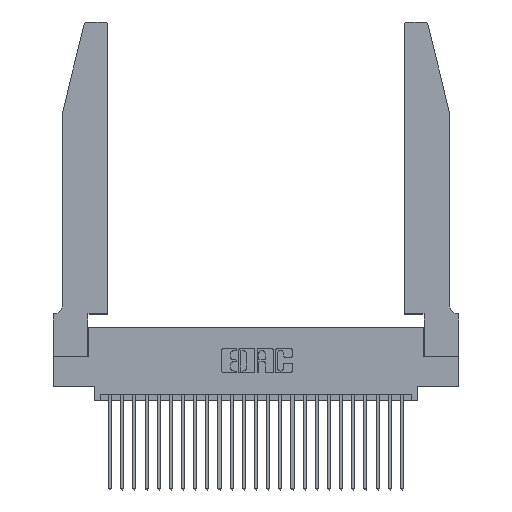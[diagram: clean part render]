
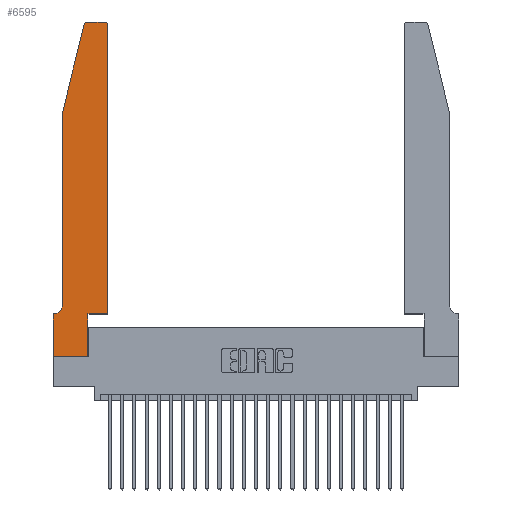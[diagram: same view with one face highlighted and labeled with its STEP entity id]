
A CAD part, top view. The second image highlights one B-rep face of the part: STEP entity #6595.
In plain terms, the highlighted planar face has unit normal (0, 0, 1).
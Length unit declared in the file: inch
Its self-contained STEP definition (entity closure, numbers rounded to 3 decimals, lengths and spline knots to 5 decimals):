
#409 = DIRECTION ( 'NONE',  ( 0., -1., 0. ) ) ;
#689 = AXIS2_PLACEMENT_3D ( 'NONE', #11758, #26268, #13857 ) ;
#794 = CARTESIAN_POINT ( 'NONE',  ( 0.0755, 2., 0.37 ) ) ;
#1211 = ORIENTED_EDGE ( 'NONE', *, *, #2643, .T. ) ;
#1948 = DIRECTION ( 'NONE',  ( 0., -1., 0. ) ) ;
#1983 = FACE_OUTER_BOUND ( 'NONE', #3229, .T. ) ;
#2109 = VERTEX_POINT ( 'NONE', #17667 ) ;
#2643 = EDGE_CURVE ( 'NONE', #11408, #11987, #24887, .T. ) ;
#2782 = AXIS2_PLACEMENT_3D ( 'NONE', #10301, #24837, #12374 ) ;
#2885 = VERTEX_POINT ( 'NONE', #21233 ) ;
#3229 = EDGE_LOOP ( 'NONE', ( #14582, #19071, #8017, #21854, #19484, #22160, #19364, #4074, #26821, #16894, #23213, #1211 ) ) ;
#3261 = AXIS2_PLACEMENT_3D ( 'NONE', #9698, #24244, #11782 ) ;
#3328 = DIRECTION ( 'NONE',  ( 0., 1., 0. ) ) ;
#4070 = CARTESIAN_POINT ( 'NONE',  ( 0.4505, 0.35, 0.37 ) ) ;
#4074 = ORIENTED_EDGE ( 'NONE', *, *, #8002, .T. ) ;
#5273 = AXIS2_PLACEMENT_3D ( 'NONE', #7003, #21202, #5955 ) ;
#5542 = EDGE_CURVE ( 'NONE', #2885, #8277, #10146, .T. ) ;
#5896 = EDGE_CURVE ( 'NONE', #8739, #23417, #7189, .T. ) ;
#5955 = DIRECTION ( 'NONE',  ( 1., 0., 0. ) ) ;
#6237 = EDGE_CURVE ( 'NONE', #8277, #13397, #14646, .T. ) ;
#6432 = CARTESIAN_POINT ( 'NONE',  ( 0.0755, 2., 0.37 ) ) ;
#6531 = VECTOR ( 'NONE', #16943, 39.37008 ) ;
#6595 = ADVANCED_FACE ( 'NONE', ( #1983 ), #20097, .T. ) ;
#6630 = CARTESIAN_POINT ( 'NONE',  ( 0.0055, 0.35, 0.37 ) ) ;
#7003 = CARTESIAN_POINT ( 'NONE',  ( 0.4205, 2.72, 0.37 ) ) ;
#7189 = LINE ( 'NONE', #19034, #6531 ) ;
#7481 = VECTOR ( 'NONE', #409, 39.37008 ) ;
#8002 = EDGE_CURVE ( 'NONE', #19930, #8739, #19979, .T. ) ;
#8017 = ORIENTED_EDGE ( 'NONE', *, *, #6237, .T. ) ;
#8058 = EDGE_CURVE ( 'NONE', #23417, #9250, #18019, .T. ) ;
#8104 = LINE ( 'NONE', #17901, #24679 ) ;
#8179 = CARTESIAN_POINT ( 'NONE',  ( 0.2605, 2.75, 0.37 ) ) ;
#8277 = VERTEX_POINT ( 'NONE', #15260 ) ;
#8739 = VERTEX_POINT ( 'NONE', #18981 ) ;
#9103 = VECTOR ( 'NONE', #21004, 39.37008 ) ;
#9250 = VERTEX_POINT ( 'NONE', #12844 ) ;
#9647 = LINE ( 'NONE', #8179, #26201 ) ;
#9698 = CARTESIAN_POINT ( 'NONE',  ( 0., 0.35, 0.37 ) ) ;
#10146 = CIRCLE ( 'NONE', #689, 0.03 ) ;
#10180 = CARTESIAN_POINT ( 'NONE',  ( 0., 0., 0.37 ) ) ;
#10301 = CARTESIAN_POINT ( 'NONE',  ( 0.0055, 0.42, 0.37 ) ) ;
#10871 = EDGE_CURVE ( 'NONE', #13397, #22568, #13611, .T. ) ;
#11057 = VECTOR ( 'NONE', #12876, 39.37008 ) ;
#11408 = VERTEX_POINT ( 'NONE', #16625 ) ;
#11758 = CARTESIAN_POINT ( 'NONE',  ( 0.284, 2.72, 0.37 ) ) ;
#11782 = DIRECTION ( 'NONE',  ( 1., 0., 0. ) ) ;
#11987 = VERTEX_POINT ( 'NONE', #12321 ) ;
#12257 = CARTESIAN_POINT ( 'NONE',  ( 0.0755, 2., 0.37 ) ) ;
#12321 = CARTESIAN_POINT ( 'NONE',  ( 0.4205, 2.75, 0.37 ) ) ;
#12374 = DIRECTION ( 'NONE',  ( -1., 0., 0. ) ) ;
#12844 = CARTESIAN_POINT ( 'NONE',  ( 0.4505, 0.35, 0.37 ) ) ;
#12876 = DIRECTION ( 'NONE',  ( -1., 0., 0. ) ) ;
#13397 = VERTEX_POINT ( 'NONE', #794 ) ;
#13611 = LINE ( 'NONE', #12257, #24033 ) ;
#13857 = DIRECTION ( 'NONE',  ( 1., 0., 0. ) ) ;
#14406 = VECTOR ( 'NONE', #22661, 39.37008 ) ;
#14582 = ORIENTED_EDGE ( 'NONE', *, *, #26098, .T. ) ;
#14646 = LINE ( 'NONE', #6432, #9103 ) ;
#15260 = CARTESIAN_POINT ( 'NONE',  ( 0.25487, 2.72718, 0.37 ) ) ;
#16625 = CARTESIAN_POINT ( 'NONE',  ( 0.4505, 2.72, 0.37 ) ) ;
#16894 = ORIENTED_EDGE ( 'NONE', *, *, #8058, .T. ) ;
#16943 = DIRECTION ( 'NONE',  ( 0., 1., 0. ) ) ;
#17103 = EDGE_CURVE ( 'NONE', #2109, #19930, #18572, .T. ) ;
#17173 = EDGE_CURVE ( 'NONE', #21925, #2109, #22156, .T. ) ;
#17176 = CARTESIAN_POINT ( 'NONE',  ( 0.0755, 0.35, 0.37 ) ) ;
#17667 = CARTESIAN_POINT ( 'NONE',  ( 0., 0.35, 0.37 ) ) ;
#17901 = CARTESIAN_POINT ( 'NONE',  ( 0.4505, 0.35, 0.37 ) ) ;
#18019 = LINE ( 'NONE', #4070, #23537 ) ;
#18154 = CARTESIAN_POINT ( 'NONE',  ( 0., 0., 0.37 ) ) ;
#18310 = EDGE_CURVE ( 'NONE', #22568, #21925, #18680, .T. ) ;
#18572 = LINE ( 'NONE', #23087, #7481 ) ;
#18680 = CIRCLE ( 'NONE', #2782, 0.07 ) ;
#18981 = CARTESIAN_POINT ( 'NONE',  ( 0.2865, 0., 0.37 ) ) ;
#19034 = CARTESIAN_POINT ( 'NONE',  ( 0.2865, 0.35, 0.37 ) ) ;
#19061 = CARTESIAN_POINT ( 'NONE',  ( 0.2865, 0.35, 0.37 ) ) ;
#19071 = ORIENTED_EDGE ( 'NONE', *, *, #5542, .T. ) ;
#19364 = ORIENTED_EDGE ( 'NONE', *, *, #17103, .T. ) ;
#19484 = ORIENTED_EDGE ( 'NONE', *, *, #18310, .T. ) ;
#19930 = VERTEX_POINT ( 'NONE', #18154 ) ;
#19979 = LINE ( 'NONE', #10180, #14406 ) ;
#20097 = PLANE ( 'NONE',  #3261 ) ;
#20403 = CARTESIAN_POINT ( 'NONE',  ( 0.0755, 0.42, 0.37 ) ) ;
#20736 = DIRECTION ( 'NONE',  ( 1., 0., 0. ) ) ;
#21004 = DIRECTION ( 'NONE',  ( -0.239, -0.971, 0. ) ) ;
#21202 = DIRECTION ( 'NONE',  ( 0., 0., 1. ) ) ;
#21233 = CARTESIAN_POINT ( 'NONE',  ( 0.284, 2.75, 0.37 ) ) ;
#21854 = ORIENTED_EDGE ( 'NONE', *, *, #10871, .T. ) ;
#21925 = VERTEX_POINT ( 'NONE', #6630 ) ;
#22156 = LINE ( 'NONE', #17176, #11057 ) ;
#22160 = ORIENTED_EDGE ( 'NONE', *, *, #17173, .T. ) ;
#22568 = VERTEX_POINT ( 'NONE', #20403 ) ;
#22661 = DIRECTION ( 'NONE',  ( 1., 0., 0. ) ) ;
#22772 = DIRECTION ( 'NONE',  ( -1., 0., 0. ) ) ;
#23087 = CARTESIAN_POINT ( 'NONE',  ( 0., 0., 0.37 ) ) ;
#23213 = ORIENTED_EDGE ( 'NONE', *, *, #24299, .T. ) ;
#23417 = VERTEX_POINT ( 'NONE', #19061 ) ;
#23537 = VECTOR ( 'NONE', #20736, 39.37008 ) ;
#24033 = VECTOR ( 'NONE', #1948, 39.37008 ) ;
#24244 = DIRECTION ( 'NONE',  ( 0., 0., 1. ) ) ;
#24299 = EDGE_CURVE ( 'NONE', #9250, #11408, #8104, .T. ) ;
#24679 = VECTOR ( 'NONE', #3328, 39.37008 ) ;
#24837 = DIRECTION ( 'NONE',  ( 0., 0., -1. ) ) ;
#24887 = CIRCLE ( 'NONE', #5273, 0.03 ) ;
#26098 = EDGE_CURVE ( 'NONE', #11987, #2885, #9647, .T. ) ;
#26201 = VECTOR ( 'NONE', #22772, 39.37008 ) ;
#26268 = DIRECTION ( 'NONE',  ( 0., 0., 1. ) ) ;
#26821 = ORIENTED_EDGE ( 'NONE', *, *, #5896, .T. ) ;
